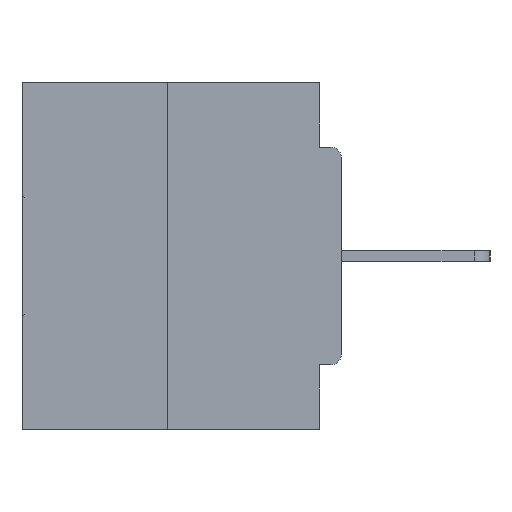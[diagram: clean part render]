
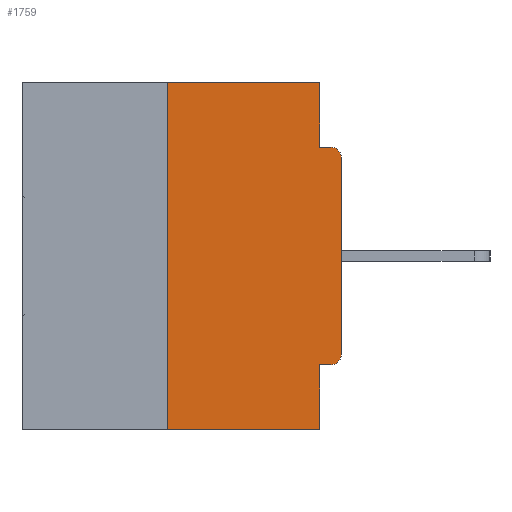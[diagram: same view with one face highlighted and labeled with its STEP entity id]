
A CAD part, left-side view. The second image highlights one B-rep face of the part: STEP entity #1759.
In plain terms, the highlighted planar face has unit normal (-1, 0, 0).
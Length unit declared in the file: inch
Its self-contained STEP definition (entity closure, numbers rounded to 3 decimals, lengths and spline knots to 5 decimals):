
#943 = VERTEX_POINT ( 'NONE', #2774 ) ;
#1136 = CARTESIAN_POINT ( 'NONE',  ( 0., 0.031, 0. ) ) ;
#1296 = EDGE_LOOP ( 'NONE', ( #2099, #3487, #17380, #13409, #25334, #9436, #4076, #8635, #30398, #17096 ) ) ;
#1759 = ADVANCED_FACE ( 'NONE', ( #15845 ), #4586, .F. ) ;
#1927 = CARTESIAN_POINT ( 'NONE',  ( 0., 0.031, 0. ) ) ;
#2001 = CARTESIAN_POINT ( 'NONE',  ( 0., 0.46, 0. ) ) ;
#2099 = ORIENTED_EDGE ( 'NONE', *, *, #19054, .F. ) ;
#2608 = VERTEX_POINT ( 'NONE', #23523 ) ;
#2774 = CARTESIAN_POINT ( 'NONE',  ( 0., 0.031, -0.0935 ) ) ;
#3209 = CARTESIAN_POINT ( 'NONE',  ( 0., 0., -0.3915 ) ) ;
#3487 = ORIENTED_EDGE ( 'NONE', *, *, #28905, .F. ) ;
#3498 = EDGE_CURVE ( 'NONE', #2608, #5211, #5980, .T. ) ;
#4076 = ORIENTED_EDGE ( 'NONE', *, *, #9860, .T. ) ;
#4097 = DIRECTION ( 'NONE',  ( 0., 0., -1. ) ) ;
#4190 = VECTOR ( 'NONE', #18034, 39.37008 ) ;
#4377 = LINE ( 'NONE', #31242, #15003 ) ;
#4586 = PLANE ( 'NONE',  #19966 ) ;
#4643 = EDGE_CURVE ( 'NONE', #16136, #6340, #4377, .T. ) ;
#5099 = LINE ( 'NONE', #12833, #18460 ) ;
#5211 = VERTEX_POINT ( 'NONE', #3209 ) ;
#5505 = CARTESIAN_POINT ( 'NONE',  ( 0., 0., 0. ) ) ;
#5980 = CIRCLE ( 'NONE', #32339, 0.015 ) ;
#6299 = LINE ( 'NONE', #33324, #4190 ) ;
#6340 = VERTEX_POINT ( 'NONE', #26651 ) ;
#6843 = CIRCLE ( 'NONE', #26501, 0.015 ) ;
#7184 = DIRECTION ( 'NONE',  ( 0., -1., 0. ) ) ;
#7393 = CARTESIAN_POINT ( 'NONE',  ( 0., 0.46, 0. ) ) ;
#7793 = LINE ( 'NONE', #5505, #33854 ) ;
#8204 = DIRECTION ( 'NONE',  ( -1., 0., 0. ) ) ;
#8545 = LINE ( 'NONE', #19123, #33670 ) ;
#8635 = ORIENTED_EDGE ( 'NONE', *, *, #32095, .T. ) ;
#9391 = VECTOR ( 'NONE', #4097, 39.37008 ) ;
#9436 = ORIENTED_EDGE ( 'NONE', *, *, #3498, .T. ) ;
#9860 = EDGE_CURVE ( 'NONE', #5211, #34400, #7793, .T. ) ;
#10422 = LINE ( 'NONE', #2001, #18472 ) ;
#12008 = CARTESIAN_POINT ( 'NONE',  ( 0., 0., -0.0935 ) ) ;
#12833 = CARTESIAN_POINT ( 'NONE',  ( 0., 0.25, 0. ) ) ;
#13409 = ORIENTED_EDGE ( 'NONE', *, *, #30594, .F. ) ;
#13831 = CARTESIAN_POINT ( 'NONE',  ( 0., 0.015, -0.3915 ) ) ;
#14928 = EDGE_CURVE ( 'NONE', #33092, #943, #22445, .T. ) ;
#15003 = VECTOR ( 'NONE', #7184, 39.37008 ) ;
#15712 = CARTESIAN_POINT ( 'NONE',  ( 0., 0.25, -0.5 ) ) ;
#15845 = FACE_OUTER_BOUND ( 'NONE', #1296, .T. ) ;
#16136 = VERTEX_POINT ( 'NONE', #15712 ) ;
#16467 = DIRECTION ( 'NONE',  ( 0., 0., -1. ) ) ;
#16848 = DIRECTION ( 'NONE',  ( 0., 0., -1. ) ) ;
#16986 = VERTEX_POINT ( 'NONE', #34392 ) ;
#17096 = ORIENTED_EDGE ( 'NONE', *, *, #14928, .F. ) ;
#17380 = ORIENTED_EDGE ( 'NONE', *, *, #4643, .T. ) ;
#17682 = EDGE_CURVE ( 'NONE', #943, #18093, #27834, .T. ) ;
#18034 = DIRECTION ( 'NONE',  ( 0., 1., 0. ) ) ;
#18093 = VERTEX_POINT ( 'NONE', #33195 ) ;
#18279 = CARTESIAN_POINT ( 'NONE',  ( 0., 0., -0.1085 ) ) ;
#18460 = VECTOR ( 'NONE', #23759, 39.37008 ) ;
#18472 = VECTOR ( 'NONE', #21182, 39.37008 ) ;
#18485 = CARTESIAN_POINT ( 'NONE',  ( 0., 0.031, -0.4065 ) ) ;
#19054 = EDGE_CURVE ( 'NONE', #16986, #33092, #10422, .T. ) ;
#19123 = CARTESIAN_POINT ( 'NONE',  ( 0., 0.031, -0.5 ) ) ;
#19497 = VECTOR ( 'NONE', #20142, 39.37008 ) ;
#19966 = AXIS2_PLACEMENT_3D ( 'NONE', #7393, #23776, #26033 ) ;
#20142 = DIRECTION ( 'NONE',  ( 0., -1., 0. ) ) ;
#21182 = DIRECTION ( 'NONE',  ( 0., -1., 0. ) ) ;
#21384 = DIRECTION ( 'NONE',  ( -1., 0., 0. ) ) ;
#21401 = EDGE_CURVE ( 'NONE', #2608, #31381, #6299, .T. ) ;
#22445 = LINE ( 'NONE', #1136, #9391 ) ;
#23523 = CARTESIAN_POINT ( 'NONE',  ( 0., 0.015, -0.4065 ) ) ;
#23759 = DIRECTION ( 'NONE',  ( 0., 0., 1. ) ) ;
#23776 = DIRECTION ( 'NONE',  ( 1., 0., 0. ) ) ;
#25334 = ORIENTED_EDGE ( 'NONE', *, *, #21401, .F. ) ;
#26033 = DIRECTION ( 'NONE',  ( 0., 0., -1. ) ) ;
#26501 = AXIS2_PLACEMENT_3D ( 'NONE', #31880, #21384, #32059 ) ;
#26651 = CARTESIAN_POINT ( 'NONE',  ( 0., 0.031, -0.5 ) ) ;
#27108 = DIRECTION ( 'NONE',  ( 0., 0., 1. ) ) ;
#27834 = LINE ( 'NONE', #12008, #19497 ) ;
#28905 = EDGE_CURVE ( 'NONE', #16136, #16986, #5099, .T. ) ;
#30398 = ORIENTED_EDGE ( 'NONE', *, *, #17682, .F. ) ;
#30594 = EDGE_CURVE ( 'NONE', #31381, #6340, #8545, .T. ) ;
#31242 = CARTESIAN_POINT ( 'NONE',  ( 0., 0.46, -0.5 ) ) ;
#31381 = VERTEX_POINT ( 'NONE', #18485 ) ;
#31880 = CARTESIAN_POINT ( 'NONE',  ( 0., 0.015, -0.1085 ) ) ;
#32059 = DIRECTION ( 'NONE',  ( 0., 0., -1. ) ) ;
#32095 = EDGE_CURVE ( 'NONE', #34400, #18093, #6843, .T. ) ;
#32339 = AXIS2_PLACEMENT_3D ( 'NONE', #13831, #8204, #16848 ) ;
#33092 = VERTEX_POINT ( 'NONE', #1927 ) ;
#33195 = CARTESIAN_POINT ( 'NONE',  ( 0., 0.015, -0.0935 ) ) ;
#33324 = CARTESIAN_POINT ( 'NONE',  ( 0., 0., -0.4065 ) ) ;
#33670 = VECTOR ( 'NONE', #16467, 39.37008 ) ;
#33854 = VECTOR ( 'NONE', #27108, 39.37008 ) ;
#34392 = CARTESIAN_POINT ( 'NONE',  ( 0., 0.25, 0. ) ) ;
#34400 = VERTEX_POINT ( 'NONE', #18279 ) ;
